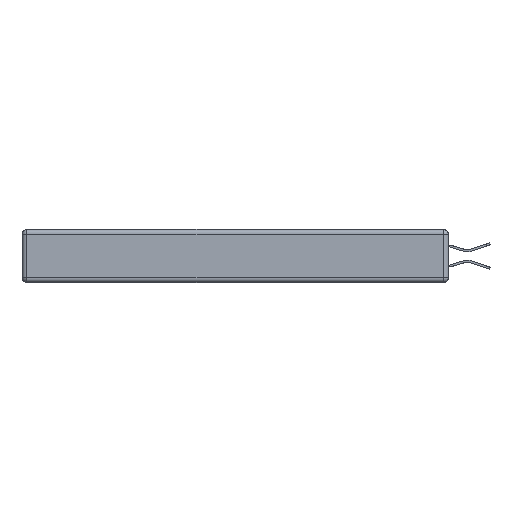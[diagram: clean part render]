
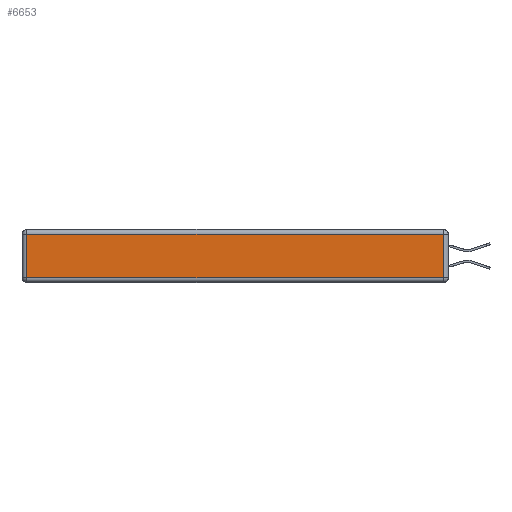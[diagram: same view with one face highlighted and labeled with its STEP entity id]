
A CAD part, left-side view. The second image highlights one B-rep face of the part: STEP entity #6653.
In plain terms, the highlighted planar face has unit normal (-1, 0, 0).
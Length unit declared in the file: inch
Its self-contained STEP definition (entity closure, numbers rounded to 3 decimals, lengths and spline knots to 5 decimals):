
#914 = EDGE_CURVE ( 'NONE', #11429, #10021, #2018, .T. ) ;
#1147 = DIRECTION ( 'NONE',  ( -1., 0., 0. ) ) ;
#1192 = ORIENTED_EDGE ( 'NONE', *, *, #914, .T. ) ;
#1525 = VERTEX_POINT ( 'NONE', #23313 ) ;
#1608 = DIRECTION ( 'NONE',  ( 0., 0., 1. ) ) ;
#2018 = LINE ( 'NONE', #25540, #14743 ) ;
#2995 = CARTESIAN_POINT ( 'NONE',  ( 0., 2.72, -0.313 ) ) ;
#3345 = LINE ( 'NONE', #17345, #20421 ) ;
#4526 = CARTESIAN_POINT ( 'NONE',  ( 0., 2.72, -0.03 ) ) ;
#5476 = DIRECTION ( 'NONE',  ( 0., 1., 0. ) ) ;
#5941 = FACE_OUTER_BOUND ( 'NONE', #13523, .T. ) ;
#6653 = ADVANCED_FACE ( 'NONE', ( #5941 ), #10074, .T. ) ;
#10021 = VERTEX_POINT ( 'NONE', #4526 ) ;
#10074 = PLANE ( 'NONE',  #21796 ) ;
#11429 = VERTEX_POINT ( 'NONE', #13368 ) ;
#12465 = VECTOR ( 'NONE', #14893, 39.37008 ) ;
#13368 = CARTESIAN_POINT ( 'NONE',  ( 0., 0.03, -0.03 ) ) ;
#13523 = EDGE_LOOP ( 'NONE', ( #26183, #25460, #1192, #20934 ) ) ;
#13562 = EDGE_CURVE ( 'NONE', #1525, #11429, #21224, .T. ) ;
#13976 = CARTESIAN_POINT ( 'NONE',  ( 0., 0., -0.343 ) ) ;
#14411 = CARTESIAN_POINT ( 'NONE',  ( 0., 0.03, -0.343 ) ) ;
#14743 = VECTOR ( 'NONE', #5476, 39.37008 ) ;
#14841 = EDGE_CURVE ( 'NONE', #10021, #26455, #19816, .T. ) ;
#14893 = DIRECTION ( 'NONE',  ( 0., 0., -1. ) ) ;
#15107 = DIRECTION ( 'NONE',  ( 0., -1., 0. ) ) ;
#15512 = VECTOR ( 'NONE', #1608, 39.37008 ) ;
#17345 = CARTESIAN_POINT ( 'NONE',  ( 0., 0., -0.313 ) ) ;
#19816 = LINE ( 'NONE', #27715, #12465 ) ;
#20421 = VECTOR ( 'NONE', #15107, 39.37008 ) ;
#20934 = ORIENTED_EDGE ( 'NONE', *, *, #14841, .T. ) ;
#21224 = LINE ( 'NONE', #14411, #15512 ) ;
#21796 = AXIS2_PLACEMENT_3D ( 'NONE', #13976, #1147, #23964 ) ;
#23313 = CARTESIAN_POINT ( 'NONE',  ( 0., 0.03, -0.313 ) ) ;
#23964 = DIRECTION ( 'NONE',  ( 0., 0., 1. ) ) ;
#25460 = ORIENTED_EDGE ( 'NONE', *, *, #13562, .T. ) ;
#25540 = CARTESIAN_POINT ( 'NONE',  ( 0., 2.75, -0.03 ) ) ;
#26183 = ORIENTED_EDGE ( 'NONE', *, *, #27502, .T. ) ;
#26455 = VERTEX_POINT ( 'NONE', #2995 ) ;
#27502 = EDGE_CURVE ( 'NONE', #26455, #1525, #3345, .T. ) ;
#27715 = CARTESIAN_POINT ( 'NONE',  ( 0., 2.72, -0.343 ) ) ;
